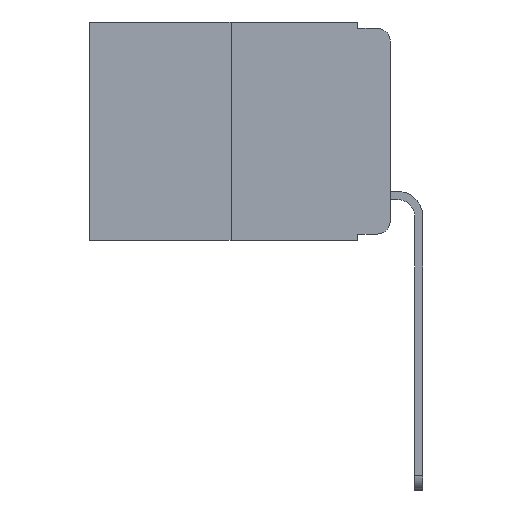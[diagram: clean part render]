
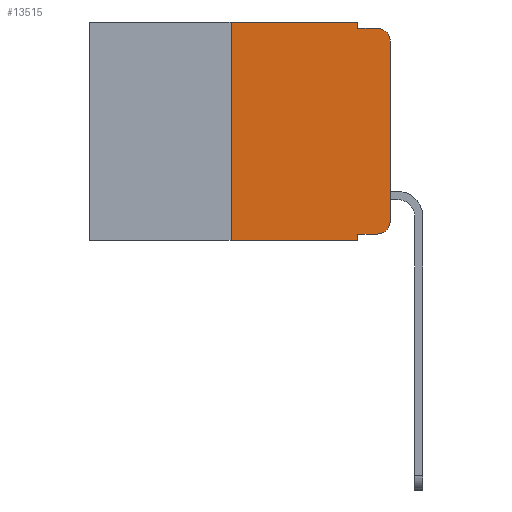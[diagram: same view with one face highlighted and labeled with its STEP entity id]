
A CAD part, left-side view. The second image highlights one B-rep face of the part: STEP entity #13515.
In plain terms, the highlighted planar face has unit normal (-1, 0, 0).
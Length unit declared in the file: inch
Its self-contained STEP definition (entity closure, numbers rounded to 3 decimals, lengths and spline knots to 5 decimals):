
#42 = ORIENTED_EDGE ( 'NONE', *, *, #2185, .F. ) ;
#410 = VERTEX_POINT ( 'NONE', #5201 ) ;
#606 = LINE ( 'NONE', #15282, #4348 ) ;
#1074 = DIRECTION ( 'NONE',  ( 0., 0., -1. ) ) ;
#1367 = VERTEX_POINT ( 'NONE', #9729 ) ;
#1543 = DIRECTION ( 'NONE',  ( 0., 0., -1. ) ) ;
#1779 = CARTESIAN_POINT ( 'NONE',  ( 0., 0.02, -0.03 ) ) ;
#2009 = ORIENTED_EDGE ( 'NONE', *, *, #13721, .T. ) ;
#2148 = CARTESIAN_POINT ( 'NONE',  ( 0., 0., -0.313 ) ) ;
#2185 = EDGE_CURVE ( 'NONE', #13835, #9236, #15392, .T. ) ;
#2526 = ORIENTED_EDGE ( 'NONE', *, *, #3339, .T. ) ;
#2700 = CARTESIAN_POINT ( 'NONE',  ( 0., 0.25, 0. ) ) ;
#3135 = VERTEX_POINT ( 'NONE', #2148 ) ;
#3167 = CARTESIAN_POINT ( 'NONE',  ( 0., 0., -0.03 ) ) ;
#3246 = FACE_OUTER_BOUND ( 'NONE', #11882, .T. ) ;
#3339 = EDGE_CURVE ( 'NONE', #1367, #7870, #3711, .T. ) ;
#3437 = CIRCLE ( 'NONE', #6504, 0.02 ) ;
#3622 = DIRECTION ( 'NONE',  ( -1., 0., 0. ) ) ;
#3711 = LINE ( 'NONE', #11030, #7088 ) ;
#3868 = VECTOR ( 'NONE', #11180, 39.37008 ) ;
#4325 = VECTOR ( 'NONE', #8536, 39.37008 ) ;
#4348 = VECTOR ( 'NONE', #8163, 39.37008 ) ;
#4392 = VECTOR ( 'NONE', #1074, 39.37008 ) ;
#4935 = EDGE_CURVE ( 'NONE', #1367, #410, #11353, .T. ) ;
#5069 = VERTEX_POINT ( 'NONE', #5171 ) ;
#5073 = ORIENTED_EDGE ( 'NONE', *, *, #7820, .T. ) ;
#5171 = CARTESIAN_POINT ( 'NONE',  ( 0., 0.25, -0.343 ) ) ;
#5201 = CARTESIAN_POINT ( 'NONE',  ( 0., 0.051, -0.343 ) ) ;
#5234 = CARTESIAN_POINT ( 'NONE',  ( 0., 0.02, -0.333 ) ) ;
#5304 = DIRECTION ( 'NONE',  ( -1., 0., 0. ) ) ;
#5530 = VERTEX_POINT ( 'NONE', #11670 ) ;
#5898 = VECTOR ( 'NONE', #9835, 39.37008 ) ;
#6294 = EDGE_CURVE ( 'NONE', #5069, #13835, #13336, .T. ) ;
#6422 = DIRECTION ( 'NONE',  ( 1., 0., 0. ) ) ;
#6504 = AXIS2_PLACEMENT_3D ( 'NONE', #1779, #5304, #8924 ) ;
#6860 = ORIENTED_EDGE ( 'NONE', *, *, #8198, .F. ) ;
#7088 = VECTOR ( 'NONE', #14526, 39.37008 ) ;
#7298 = CIRCLE ( 'NONE', #9441, 0.02 ) ;
#7529 = CARTESIAN_POINT ( 'NONE',  ( 0., 0.473, 0. ) ) ;
#7820 = EDGE_CURVE ( 'NONE', #7870, #3135, #7298, .T. ) ;
#7870 = VERTEX_POINT ( 'NONE', #5234 ) ;
#8163 = DIRECTION ( 'NONE',  ( 0., -1., 0. ) ) ;
#8198 = EDGE_CURVE ( 'NONE', #9236, #13676, #12184, .T. ) ;
#8281 = CARTESIAN_POINT ( 'NONE',  ( 0., 0.051, 0. ) ) ;
#8435 = DIRECTION ( 'NONE',  ( 0., 0., -1. ) ) ;
#8536 = DIRECTION ( 'NONE',  ( 0., 0., 1. ) ) ;
#8641 = CARTESIAN_POINT ( 'NONE',  ( 0., 0.473, 0. ) ) ;
#8924 = DIRECTION ( 'NONE',  ( 0., 0., -1. ) ) ;
#9179 = VECTOR ( 'NONE', #14720, 39.37008 ) ;
#9236 = VERTEX_POINT ( 'NONE', #10813 ) ;
#9441 = AXIS2_PLACEMENT_3D ( 'NONE', #13150, #3622, #8435 ) ;
#9729 = CARTESIAN_POINT ( 'NONE',  ( 0., 0.051, -0.333 ) ) ;
#9768 = ORIENTED_EDGE ( 'NONE', *, *, #10060, .F. ) ;
#9784 = CARTESIAN_POINT ( 'NONE',  ( 0., 0., 0. ) ) ;
#9835 = DIRECTION ( 'NONE',  ( 0., 0., 1. ) ) ;
#9932 = DIRECTION ( 'NONE',  ( 0., 0., -1. ) ) ;
#10045 = LINE ( 'NONE', #13628, #3868 ) ;
#10060 = EDGE_CURVE ( 'NONE', #13676, #5530, #10045, .T. ) ;
#10462 = EDGE_CURVE ( 'NONE', #3135, #15301, #14719, .T. ) ;
#10813 = CARTESIAN_POINT ( 'NONE',  ( 0., 0.051, 0. ) ) ;
#11030 = CARTESIAN_POINT ( 'NONE',  ( 0., 0.051, -0.333 ) ) ;
#11180 = DIRECTION ( 'NONE',  ( 0., -1., 0. ) ) ;
#11353 = LINE ( 'NONE', #8281, #4392 ) ;
#11563 = CARTESIAN_POINT ( 'NONE',  ( 0., 0.25, 0. ) ) ;
#11670 = CARTESIAN_POINT ( 'NONE',  ( 0., 0.02, -0.01 ) ) ;
#11882 = EDGE_LOOP ( 'NONE', ( #12229, #2009, #9768, #6860, #42, #14124, #14993, #15413, #2526, #5073 ) ) ;
#12184 = LINE ( 'NONE', #13439, #14996 ) ;
#12229 = ORIENTED_EDGE ( 'NONE', *, *, #10462, .T. ) ;
#12340 = AXIS2_PLACEMENT_3D ( 'NONE', #7529, #6422, #9932 ) ;
#13150 = CARTESIAN_POINT ( 'NONE',  ( 0., 0.02, -0.313 ) ) ;
#13336 = LINE ( 'NONE', #2700, #4325 ) ;
#13439 = CARTESIAN_POINT ( 'NONE',  ( 0., 0.051, 0. ) ) ;
#13515 = ADVANCED_FACE ( 'NONE', ( #3246 ), #14804, .F. ) ;
#13628 = CARTESIAN_POINT ( 'NONE',  ( 0., 0.051, -0.01 ) ) ;
#13676 = VERTEX_POINT ( 'NONE', #14970 ) ;
#13721 = EDGE_CURVE ( 'NONE', #15301, #5530, #3437, .T. ) ;
#13835 = VERTEX_POINT ( 'NONE', #11563 ) ;
#13848 = EDGE_CURVE ( 'NONE', #5069, #410, #606, .T. ) ;
#14124 = ORIENTED_EDGE ( 'NONE', *, *, #6294, .F. ) ;
#14526 = DIRECTION ( 'NONE',  ( 0., -1., 0. ) ) ;
#14719 = LINE ( 'NONE', #9784, #5898 ) ;
#14720 = DIRECTION ( 'NONE',  ( 0., -1., 0. ) ) ;
#14804 = PLANE ( 'NONE',  #12340 ) ;
#14970 = CARTESIAN_POINT ( 'NONE',  ( 0., 0.051, -0.01 ) ) ;
#14993 = ORIENTED_EDGE ( 'NONE', *, *, #13848, .T. ) ;
#14996 = VECTOR ( 'NONE', #1543, 39.37008 ) ;
#15282 = CARTESIAN_POINT ( 'NONE',  ( 0., 0.473, -0.343 ) ) ;
#15301 = VERTEX_POINT ( 'NONE', #3167 ) ;
#15392 = LINE ( 'NONE', #8641, #9179 ) ;
#15413 = ORIENTED_EDGE ( 'NONE', *, *, #4935, .F. ) ;
